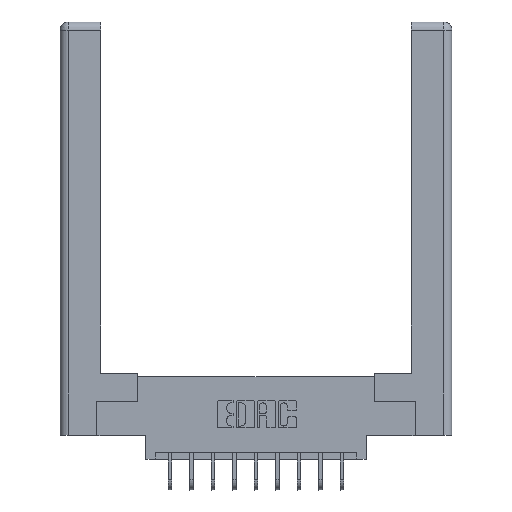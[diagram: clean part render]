
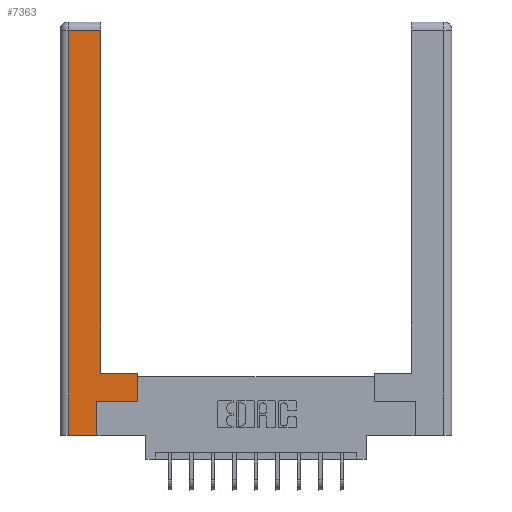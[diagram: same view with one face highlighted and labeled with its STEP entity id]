
A CAD part, top view. The second image highlights one B-rep face of the part: STEP entity #7363.
In plain terms, the highlighted planar face has unit normal (0, 0, 1).
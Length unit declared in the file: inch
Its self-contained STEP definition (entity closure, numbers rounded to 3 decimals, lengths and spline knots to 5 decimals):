
#106 = EDGE_CURVE ( 'NONE', #5633, #6737, #8729, .T. ) ;
#454 = VERTEX_POINT ( 'NONE', #2061 ) ;
#515 = EDGE_CURVE ( 'NONE', #6737, #5802, #5474, .T. ) ;
#559 = LINE ( 'NONE', #3756, #6691 ) ;
#614 = CARTESIAN_POINT ( 'NONE',  ( 0.565, 0.45, 0. ) ) ;
#621 = EDGE_CURVE ( 'NONE', #6138, #1133, #7748, .T. ) ;
#989 = LINE ( 'NONE', #13192, #8439 ) ;
#1133 = VERTEX_POINT ( 'NONE', #9956 ) ;
#1219 = ORIENTED_EDGE ( 'NONE', *, *, #515, .T. ) ;
#1542 = EDGE_LOOP ( 'NONE', ( #3461, #6589, #2927, #1219, #14320, #10092, #7345, #2856 ) ) ;
#1825 = FACE_OUTER_BOUND ( 'NONE', #1542, .T. ) ;
#2004 = DIRECTION ( 'NONE',  ( 0., 1., 0. ) ) ;
#2061 = CARTESIAN_POINT ( 'NONE',  ( 0.265, 0.245, 0. ) ) ;
#2265 = DIRECTION ( 'NONE',  ( 0., 0., -1. ) ) ;
#2371 = DIRECTION ( 'NONE',  ( -1., 0., 0. ) ) ;
#2377 = PLANE ( 'NONE',  #10705 ) ;
#2402 = CARTESIAN_POINT ( 'NONE',  ( 0.295, 2.94, 0. ) ) ;
#2417 = EDGE_CURVE ( 'NONE', #15342, #6138, #989, .T. ) ;
#2464 = DIRECTION ( 'NONE',  ( -1., 0., 0. ) ) ;
#2820 = DIRECTION ( 'NONE',  ( 0., -1., 0. ) ) ;
#2856 = ORIENTED_EDGE ( 'NONE', *, *, #621, .T. ) ;
#2927 = ORIENTED_EDGE ( 'NONE', *, *, #106, .T. ) ;
#2946 = VECTOR ( 'NONE', #2371, 39.37008 ) ;
#3119 = EDGE_CURVE ( 'NONE', #5802, #454, #13037, .T. ) ;
#3200 = VECTOR ( 'NONE', #2464, 39.37008 ) ;
#3461 = ORIENTED_EDGE ( 'NONE', *, *, #5181, .T. ) ;
#3756 = CARTESIAN_POINT ( 'NONE',  ( 0.295, 3., 0. ) ) ;
#3759 = EDGE_CURVE ( 'NONE', #454, #15342, #9003, .T. ) ;
#4209 = VECTOR ( 'NONE', #13542, 39.37008 ) ;
#4889 = DIRECTION ( 'NONE',  ( 0., 1., 0. ) ) ;
#5181 = EDGE_CURVE ( 'NONE', #1133, #10852, #559, .T. ) ;
#5340 = CARTESIAN_POINT ( 'NONE',  ( 0.0615, 2.94, 0. ) ) ;
#5474 = LINE ( 'NONE', #8311, #13124 ) ;
#5484 = VECTOR ( 'NONE', #2820, 39.37008 ) ;
#5633 = VERTEX_POINT ( 'NONE', #5340 ) ;
#5802 = VERTEX_POINT ( 'NONE', #7945 ) ;
#6138 = VERTEX_POINT ( 'NONE', #614 ) ;
#6589 = ORIENTED_EDGE ( 'NONE', *, *, #13270, .T. ) ;
#6691 = VECTOR ( 'NONE', #4889, 39.37008 ) ;
#6737 = VERTEX_POINT ( 'NONE', #15121 ) ;
#7100 = CARTESIAN_POINT ( 'NONE',  ( 0.295, 0.45, 0. ) ) ;
#7345 = ORIENTED_EDGE ( 'NONE', *, *, #2417, .T. ) ;
#7363 = ADVANCED_FACE ( 'NONE', ( #1825 ), #2377, .F. ) ;
#7421 = CARTESIAN_POINT ( 'NONE',  ( 0.565, 0.245, 0. ) ) ;
#7748 = LINE ( 'NONE', #7100, #2946 ) ;
#7764 = DIRECTION ( 'NONE',  ( 1., 0., 0. ) ) ;
#7945 = CARTESIAN_POINT ( 'NONE',  ( 0.265, 0., 0. ) ) ;
#8311 = CARTESIAN_POINT ( 'NONE',  ( 0.265, 0., 0. ) ) ;
#8439 = VECTOR ( 'NONE', #2004, 39.37008 ) ;
#8729 = LINE ( 'NONE', #10152, #5484 ) ;
#9003 = LINE ( 'NONE', #15180, #15661 ) ;
#9797 = CARTESIAN_POINT ( 'NONE',  ( 0.0615, 2.94, 0. ) ) ;
#9956 = CARTESIAN_POINT ( 'NONE',  ( 0.295, 0.45, 0. ) ) ;
#10092 = ORIENTED_EDGE ( 'NONE', *, *, #3759, .T. ) ;
#10152 = CARTESIAN_POINT ( 'NONE',  ( 0.0615, 0., 0. ) ) ;
#10705 = AXIS2_PLACEMENT_3D ( 'NONE', #10935, #2265, #15674 ) ;
#10852 = VERTEX_POINT ( 'NONE', #2402 ) ;
#10935 = CARTESIAN_POINT ( 'NONE',  ( 0., 0., 0. ) ) ;
#11067 = CARTESIAN_POINT ( 'NONE',  ( 0.265, 0.245, 0. ) ) ;
#13037 = LINE ( 'NONE', #11067, #4209 ) ;
#13124 = VECTOR ( 'NONE', #13198, 39.37008 ) ;
#13192 = CARTESIAN_POINT ( 'NONE',  ( 0.565, 0.45, 0. ) ) ;
#13198 = DIRECTION ( 'NONE',  ( 1., 0., 0. ) ) ;
#13270 = EDGE_CURVE ( 'NONE', #10852, #5633, #14505, .T. ) ;
#13542 = DIRECTION ( 'NONE',  ( 0., 1., 0. ) ) ;
#14320 = ORIENTED_EDGE ( 'NONE', *, *, #3119, .T. ) ;
#14505 = LINE ( 'NONE', #9797, #3200 ) ;
#15121 = CARTESIAN_POINT ( 'NONE',  ( 0.0615, 0., 0. ) ) ;
#15180 = CARTESIAN_POINT ( 'NONE',  ( 0.565, 0.245, 0. ) ) ;
#15342 = VERTEX_POINT ( 'NONE', #7421 ) ;
#15661 = VECTOR ( 'NONE', #7764, 39.37008 ) ;
#15674 = DIRECTION ( 'NONE',  ( -1., 0., 0. ) ) ;
